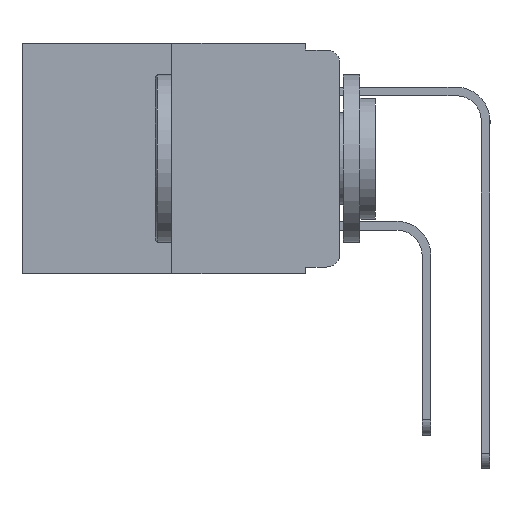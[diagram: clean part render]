
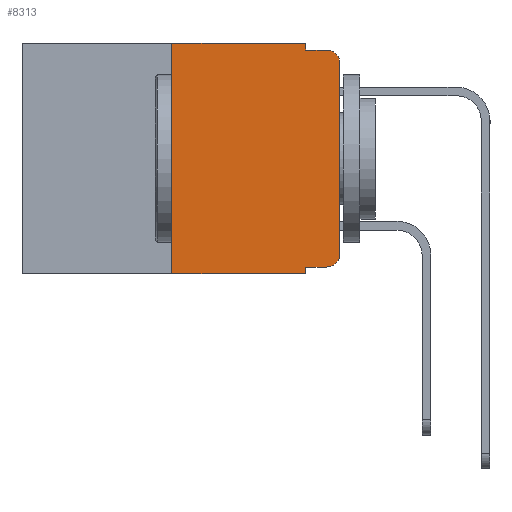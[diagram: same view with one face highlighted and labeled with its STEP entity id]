
A CAD part, left-side view. The second image highlights one B-rep face of the part: STEP entity #8313.
In plain terms, the highlighted planar face has unit normal (-1, 0, 0).
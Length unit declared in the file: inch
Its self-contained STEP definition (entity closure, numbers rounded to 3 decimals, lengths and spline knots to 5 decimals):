
#473 = DIRECTION ( 'NONE',  ( 0., 0., -1. ) ) ;
#631 = ORIENTED_EDGE ( 'NONE', *, *, #1014, .F. ) ;
#1014 = EDGE_CURVE ( 'NONE', #20621, #9250, #21823, .T. ) ;
#2467 = DIRECTION ( 'NONE',  ( 0., 0., -1. ) ) ;
#2662 = DIRECTION ( 'NONE',  ( 0., 0., 1. ) ) ;
#3067 = EDGE_CURVE ( 'NONE', #3556, #21797, #6467, .T. ) ;
#3164 = VECTOR ( 'NONE', #14031, 39.37008 ) ;
#3176 = ORIENTED_EDGE ( 'NONE', *, *, #12998, .T. ) ;
#3477 = ORIENTED_EDGE ( 'NONE', *, *, #6834, .F. ) ;
#3556 = VERTEX_POINT ( 'NONE', #13684 ) ;
#3874 = CARTESIAN_POINT ( 'NONE',  ( 0., 0.051, 0. ) ) ;
#4014 = AXIS2_PLACEMENT_3D ( 'NONE', #5642, #6668, #6766 ) ;
#4340 = EDGE_CURVE ( 'NONE', #17855, #3556, #17456, .T. ) ;
#4405 = CARTESIAN_POINT ( 'NONE',  ( 0., 0.051, 0. ) ) ;
#5200 = VECTOR ( 'NONE', #2467, 39.37008 ) ;
#5599 = EDGE_CURVE ( 'NONE', #17855, #6451, #20012, .T. ) ;
#5642 = CARTESIAN_POINT ( 'NONE',  ( 0., 0.02, -0.313 ) ) ;
#5700 = VERTEX_POINT ( 'NONE', #23034 ) ;
#6005 = DIRECTION ( 'NONE',  ( 0., -1., 0. ) ) ;
#6451 = VERTEX_POINT ( 'NONE', #18062 ) ;
#6467 = CIRCLE ( 'NONE', #4014, 0.02 ) ;
#6668 = DIRECTION ( 'NONE',  ( -1., 0., 0. ) ) ;
#6723 = ORIENTED_EDGE ( 'NONE', *, *, #3067, .T. ) ;
#6766 = DIRECTION ( 'NONE',  ( 0., 0., -1. ) ) ;
#6834 = EDGE_CURVE ( 'NONE', #20053, #20621, #9809, .T. ) ;
#7587 = ORIENTED_EDGE ( 'NONE', *, *, #5599, .F. ) ;
#7608 = LINE ( 'NONE', #12171, #16917 ) ;
#8107 = EDGE_CURVE ( 'NONE', #9250, #5700, #7608, .T. ) ;
#8249 = CARTESIAN_POINT ( 'NONE',  ( 0., 0.25, 0. ) ) ;
#8313 = ADVANCED_FACE ( 'NONE', ( #12758 ), #16872, .F. ) ;
#8327 = CIRCLE ( 'NONE', #18058, 0.02 ) ;
#8652 = VECTOR ( 'NONE', #2662, 39.37008 ) ;
#8992 = CARTESIAN_POINT ( 'NONE',  ( 0., 0., -0.03 ) ) ;
#9250 = VERTEX_POINT ( 'NONE', #3874 ) ;
#9348 = EDGE_CURVE ( 'NONE', #5700, #20522, #15382, .T. ) ;
#9400 = CARTESIAN_POINT ( 'NONE',  ( 0., 0.473, 0. ) ) ;
#9476 = DIRECTION ( 'NONE',  ( 1., 0., 0. ) ) ;
#9809 = LINE ( 'NONE', #19472, #8652 ) ;
#9841 = VECTOR ( 'NONE', #11941, 39.37008 ) ;
#10041 = CARTESIAN_POINT ( 'NONE',  ( 0., 0.051, -0.333 ) ) ;
#10176 = CARTESIAN_POINT ( 'NONE',  ( 0., 0.473, -0.343 ) ) ;
#10241 = CARTESIAN_POINT ( 'NONE',  ( 0., 0.25, -0.343 ) ) ;
#10514 = ORIENTED_EDGE ( 'NONE', *, *, #4340, .T. ) ;
#11331 = EDGE_LOOP ( 'NONE', ( #3176, #21445, #20629, #23613, #631, #3477, #23587, #7587, #10514, #6723 ) ) ;
#11765 = EDGE_CURVE ( 'NONE', #16512, #20522, #8327, .T. ) ;
#11836 = DIRECTION ( 'NONE',  ( -1., 0., 0. ) ) ;
#11941 = DIRECTION ( 'NONE',  ( 0., -1., 0. ) ) ;
#12171 = CARTESIAN_POINT ( 'NONE',  ( 0., 0.051, 0. ) ) ;
#12529 = CARTESIAN_POINT ( 'NONE',  ( 0., 0., 0. ) ) ;
#12758 = FACE_OUTER_BOUND ( 'NONE', #11331, .T. ) ;
#12998 = EDGE_CURVE ( 'NONE', #21797, #16512, #14299, .T. ) ;
#13684 = CARTESIAN_POINT ( 'NONE',  ( 0., 0.02, -0.333 ) ) ;
#14031 = DIRECTION ( 'NONE',  ( 0., -1., 0. ) ) ;
#14046 = DIRECTION ( 'NONE',  ( 0., 0., -1. ) ) ;
#14299 = LINE ( 'NONE', #12529, #23391 ) ;
#14428 = DIRECTION ( 'NONE',  ( 0., 0., 1. ) ) ;
#14524 = CARTESIAN_POINT ( 'NONE',  ( 0., 0.051, -0.333 ) ) ;
#14779 = VECTOR ( 'NONE', #6005, 39.37008 ) ;
#15235 = CARTESIAN_POINT ( 'NONE',  ( 0., 0.051, -0.01 ) ) ;
#15326 = LINE ( 'NONE', #10176, #9841 ) ;
#15382 = LINE ( 'NONE', #15235, #14779 ) ;
#16512 = VERTEX_POINT ( 'NONE', #8992 ) ;
#16817 = CARTESIAN_POINT ( 'NONE',  ( 0., 0., -0.313 ) ) ;
#16872 = PLANE ( 'NONE',  #19826 ) ;
#16917 = VECTOR ( 'NONE', #14046, 39.37008 ) ;
#17013 = VECTOR ( 'NONE', #20415, 39.37008 ) ;
#17266 = CARTESIAN_POINT ( 'NONE',  ( 0., 0.02, -0.01 ) ) ;
#17456 = LINE ( 'NONE', #14524, #3164 ) ;
#17603 = EDGE_CURVE ( 'NONE', #20053, #6451, #15326, .T. ) ;
#17855 = VERTEX_POINT ( 'NONE', #10041 ) ;
#18058 = AXIS2_PLACEMENT_3D ( 'NONE', #22815, #11836, #473 ) ;
#18062 = CARTESIAN_POINT ( 'NONE',  ( 0., 0.051, -0.343 ) ) ;
#19472 = CARTESIAN_POINT ( 'NONE',  ( 0., 0.25, 0. ) ) ;
#19826 = AXIS2_PLACEMENT_3D ( 'NONE', #9400, #9476, #22301 ) ;
#20012 = LINE ( 'NONE', #4405, #5200 ) ;
#20053 = VERTEX_POINT ( 'NONE', #10241 ) ;
#20415 = DIRECTION ( 'NONE',  ( 0., -1., 0. ) ) ;
#20470 = CARTESIAN_POINT ( 'NONE',  ( 0., 0.473, 0. ) ) ;
#20522 = VERTEX_POINT ( 'NONE', #17266 ) ;
#20621 = VERTEX_POINT ( 'NONE', #8249 ) ;
#20629 = ORIENTED_EDGE ( 'NONE', *, *, #9348, .F. ) ;
#21445 = ORIENTED_EDGE ( 'NONE', *, *, #11765, .T. ) ;
#21797 = VERTEX_POINT ( 'NONE', #16817 ) ;
#21823 = LINE ( 'NONE', #20470, #17013 ) ;
#22301 = DIRECTION ( 'NONE',  ( 0., 0., -1. ) ) ;
#22815 = CARTESIAN_POINT ( 'NONE',  ( 0., 0.02, -0.03 ) ) ;
#23034 = CARTESIAN_POINT ( 'NONE',  ( 0., 0.051, -0.01 ) ) ;
#23391 = VECTOR ( 'NONE', #14428, 39.37008 ) ;
#23587 = ORIENTED_EDGE ( 'NONE', *, *, #17603, .T. ) ;
#23613 = ORIENTED_EDGE ( 'NONE', *, *, #8107, .F. ) ;
